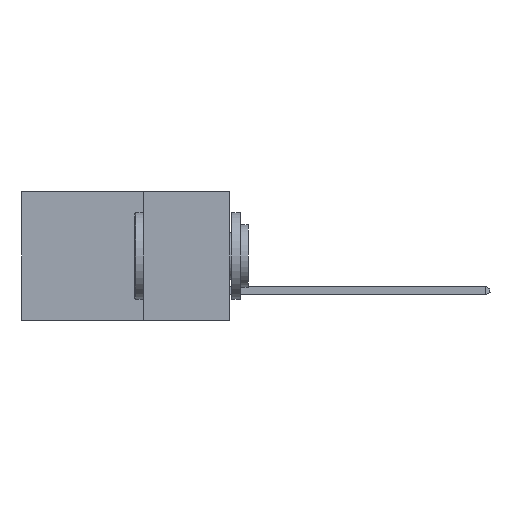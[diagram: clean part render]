
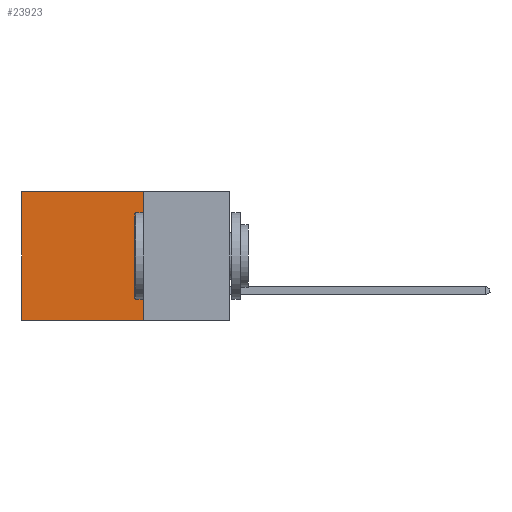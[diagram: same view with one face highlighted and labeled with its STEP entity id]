
A CAD part, left-side view. The second image highlights one B-rep face of the part: STEP entity #23923.
In plain terms, the highlighted planar face has unit normal (-1, 0, 0).
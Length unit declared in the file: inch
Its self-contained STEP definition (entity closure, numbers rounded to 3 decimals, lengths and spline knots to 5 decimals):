
#511 = EDGE_CURVE ( 'NONE', #24209, #8361, #21820, .T. ) ;
#584 = VECTOR ( 'NONE', #23602, 39.37008 ) ;
#1109 = EDGE_CURVE ( 'NONE', #16711, #8361, #23134, .T. ) ;
#1583 = CARTESIAN_POINT ( 'NONE',  ( 0.298, 0.25, -0.37 ) ) ;
#1857 = CARTESIAN_POINT ( 'NONE',  ( 0.298, 0.25, 0. ) ) ;
#2109 = EDGE_LOOP ( 'NONE', ( #5255, #23638, #25142, #15538 ) ) ;
#2116 = DIRECTION ( 'NONE',  ( 0., 1., 0. ) ) ;
#3511 = VECTOR ( 'NONE', #11995, 39.37008 ) ;
#4450 = CARTESIAN_POINT ( 'NONE',  ( 0.298, 0.25, 0. ) ) ;
#4739 = PLANE ( 'NONE',  #23530 ) ;
#5185 = EDGE_CURVE ( 'NONE', #8760, #24209, #27255, .T. ) ;
#5255 = ORIENTED_EDGE ( 'NONE', *, *, #1109, .T. ) ;
#8361 = VERTEX_POINT ( 'NONE', #21090 ) ;
#8760 = VERTEX_POINT ( 'NONE', #26416 ) ;
#11899 = EDGE_CURVE ( 'NONE', #8760, #16711, #12886, .T. ) ;
#11995 = DIRECTION ( 'NONE',  ( 0., 0., -1. ) ) ;
#12317 = CARTESIAN_POINT ( 'NONE',  ( 0.298, 0.25, -0.37 ) ) ;
#12886 = LINE ( 'NONE', #1857, #17906 ) ;
#15146 = CARTESIAN_POINT ( 'NONE',  ( 0.298, 0.25, 0. ) ) ;
#15538 = ORIENTED_EDGE ( 'NONE', *, *, #11899, .T. ) ;
#16711 = VERTEX_POINT ( 'NONE', #26786 ) ;
#17906 = VECTOR ( 'NONE', #2116, 39.37008 ) ;
#18943 = DIRECTION ( 'NONE',  ( 0., 1., 0. ) ) ;
#19163 = VECTOR ( 'NONE', #18943, 39.37008 ) ;
#20114 = CARTESIAN_POINT ( 'NONE',  ( 0.298, 0.6, 0. ) ) ;
#21090 = CARTESIAN_POINT ( 'NONE',  ( 0.298, 0.6, -0.37 ) ) ;
#21820 = LINE ( 'NONE', #1583, #19163 ) ;
#23134 = LINE ( 'NONE', #20114, #3511 ) ;
#23530 = AXIS2_PLACEMENT_3D ( 'NONE', #15146, #26066, #23714 ) ;
#23602 = DIRECTION ( 'NONE',  ( 0., 0., -1. ) ) ;
#23638 = ORIENTED_EDGE ( 'NONE', *, *, #511, .F. ) ;
#23714 = DIRECTION ( 'NONE',  ( 0., 0., -1. ) ) ;
#23923 = ADVANCED_FACE ( 'NONE', ( #24616 ), #4739, .F. ) ;
#24209 = VERTEX_POINT ( 'NONE', #12317 ) ;
#24616 = FACE_OUTER_BOUND ( 'NONE', #2109, .T. ) ;
#25142 = ORIENTED_EDGE ( 'NONE', *, *, #5185, .F. ) ;
#26066 = DIRECTION ( 'NONE',  ( 1., 0., 0. ) ) ;
#26416 = CARTESIAN_POINT ( 'NONE',  ( 0.298, 0.25, 0. ) ) ;
#26786 = CARTESIAN_POINT ( 'NONE',  ( 0.298, 0.6, 0. ) ) ;
#27255 = LINE ( 'NONE', #4450, #584 ) ;
